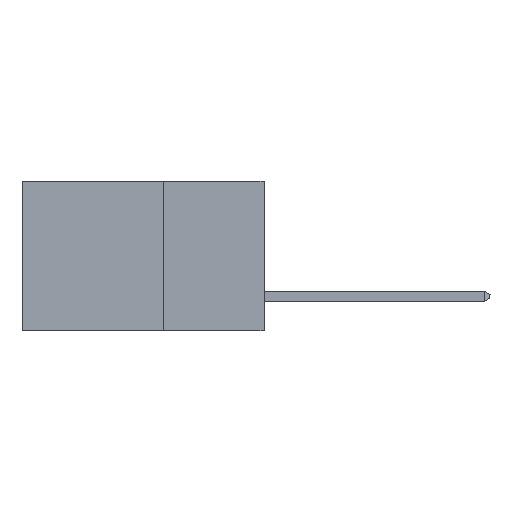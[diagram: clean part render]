
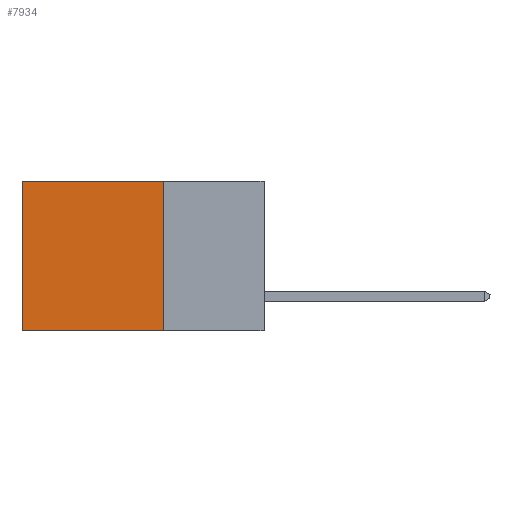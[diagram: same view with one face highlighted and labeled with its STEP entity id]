
A CAD part, left-side view. The second image highlights one B-rep face of the part: STEP entity #7934.
In plain terms, the highlighted planar face has unit normal (-1, 0, 0).
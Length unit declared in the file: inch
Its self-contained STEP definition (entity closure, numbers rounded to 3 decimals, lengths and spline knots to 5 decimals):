
#217 = VECTOR ( 'NONE', #17427, 39.37008 ) ;
#850 = DIRECTION ( 'NONE',  ( 0., 0., -1. ) ) ;
#1464 = LINE ( 'NONE', #11045, #217 ) ;
#1472 = VERTEX_POINT ( 'NONE', #6919 ) ;
#2337 = PLANE ( 'NONE',  #7391 ) ;
#2512 = EDGE_LOOP ( 'NONE', ( #9273, #8841, #13589, #15488 ) ) ;
#3160 = EDGE_CURVE ( 'NONE', #5353, #18109, #14111, .T. ) ;
#5353 = VERTEX_POINT ( 'NONE', #19306 ) ;
#5770 = FACE_OUTER_BOUND ( 'NONE', #2512, .T. ) ;
#6185 = CARTESIAN_POINT ( 'NONE',  ( 0.2615, 0.25, 0. ) ) ;
#6919 = CARTESIAN_POINT ( 'NONE',  ( 0.2615, 0.25, -0.37 ) ) ;
#7391 = AXIS2_PLACEMENT_3D ( 'NONE', #16952, #9007, #8694 ) ;
#7934 = ADVANCED_FACE ( 'NONE', ( #5770 ), #2337, .F. ) ;
#8213 = VECTOR ( 'NONE', #17368, 39.37008 ) ;
#8260 = CARTESIAN_POINT ( 'NONE',  ( 0.2615, 0.25, -0.37 ) ) ;
#8694 = DIRECTION ( 'NONE',  ( 0., 0., -1. ) ) ;
#8841 = ORIENTED_EDGE ( 'NONE', *, *, #17181, .F. ) ;
#9007 = DIRECTION ( 'NONE',  ( 1., 0., 0. ) ) ;
#9237 = VERTEX_POINT ( 'NONE', #18941 ) ;
#9273 = ORIENTED_EDGE ( 'NONE', *, *, #13333, .T. ) ;
#11045 = CARTESIAN_POINT ( 'NONE',  ( 0.2615, 0.25, -0.37 ) ) ;
#12996 = CARTESIAN_POINT ( 'NONE',  ( 0.2615, 0.6, 0. ) ) ;
#13045 = LINE ( 'NONE', #8260, #13888 ) ;
#13333 = EDGE_CURVE ( 'NONE', #18109, #9237, #13772, .T. ) ;
#13589 = ORIENTED_EDGE ( 'NONE', *, *, #16233, .F. ) ;
#13772 = LINE ( 'NONE', #20150, #15125 ) ;
#13888 = VECTOR ( 'NONE', #18167, 39.37008 ) ;
#14111 = LINE ( 'NONE', #6185, #8213 ) ;
#15125 = VECTOR ( 'NONE', #850, 39.37008 ) ;
#15488 = ORIENTED_EDGE ( 'NONE', *, *, #3160, .T. ) ;
#16233 = EDGE_CURVE ( 'NONE', #5353, #1472, #1464, .T. ) ;
#16952 = CARTESIAN_POINT ( 'NONE',  ( 0.2615, 0.25, -0.37 ) ) ;
#17181 = EDGE_CURVE ( 'NONE', #1472, #9237, #13045, .T. ) ;
#17368 = DIRECTION ( 'NONE',  ( 0., 1., 0. ) ) ;
#17427 = DIRECTION ( 'NONE',  ( 0., 0., -1. ) ) ;
#18109 = VERTEX_POINT ( 'NONE', #12996 ) ;
#18167 = DIRECTION ( 'NONE',  ( 0., 1., 0. ) ) ;
#18941 = CARTESIAN_POINT ( 'NONE',  ( 0.2615, 0.6, -0.37 ) ) ;
#19306 = CARTESIAN_POINT ( 'NONE',  ( 0.2615, 0.25, 0. ) ) ;
#20150 = CARTESIAN_POINT ( 'NONE',  ( 0.2615, 0.6, -0.37 ) ) ;
